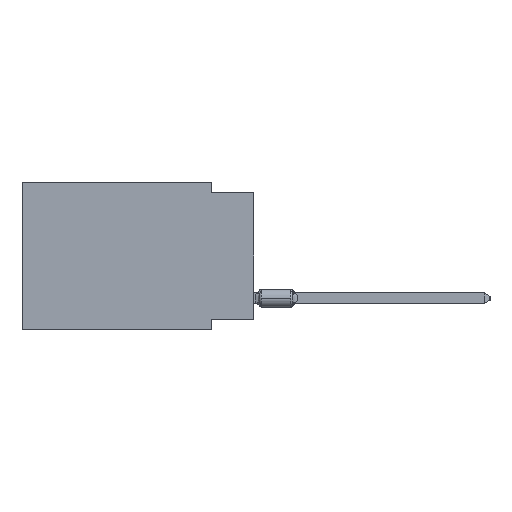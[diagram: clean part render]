
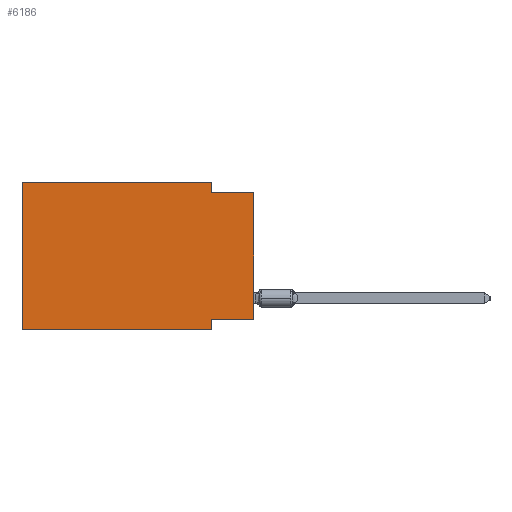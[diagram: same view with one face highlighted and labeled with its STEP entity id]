
A CAD part, left-side view. The second image highlights one B-rep face of the part: STEP entity #6186.
In plain terms, the highlighted planar face has unit normal (-1, 0, 0).
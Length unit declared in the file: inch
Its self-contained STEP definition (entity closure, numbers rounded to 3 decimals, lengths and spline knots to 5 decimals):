
#2592 = CARTESIAN_POINT ( 'NONE',  ( 0., 0.1, 0. ) ) ;
#2606 = ORIENTED_EDGE ( 'NONE', *, *, #16428, .T. ) ;
#2696 = EDGE_LOOP ( 'NONE', ( #2606, #30905, #3369, #40720, #10590, #12407, #20386, #7470 ) ) ;
#2718 = CARTESIAN_POINT ( 'NONE',  ( 0., 0.55, 0. ) ) ;
#2725 = VERTEX_POINT ( 'NONE', #41874 ) ;
#3369 = ORIENTED_EDGE ( 'NONE', *, *, #33779, .F. ) ;
#3439 = CARTESIAN_POINT ( 'NONE',  ( 0., 0., -0.325 ) ) ;
#3729 = CARTESIAN_POINT ( 'NONE',  ( 0., 0.55, 0. ) ) ;
#4168 = CARTESIAN_POINT ( 'NONE',  ( 0., 0.55, 0. ) ) ;
#6186 = ADVANCED_FACE ( 'NONE', ( #16528 ), #30312, .F. ) ;
#7351 = DIRECTION ( 'NONE',  ( 1., 0., 0. ) ) ;
#7470 = ORIENTED_EDGE ( 'NONE', *, *, #14924, .F. ) ;
#8074 = VERTEX_POINT ( 'NONE', #2592 ) ;
#10346 = DIRECTION ( 'NONE',  ( 0., 0., -1. ) ) ;
#10590 = ORIENTED_EDGE ( 'NONE', *, *, #40775, .F. ) ;
#11443 = DIRECTION ( 'NONE',  ( 0., -1., 0. ) ) ;
#11640 = VECTOR ( 'NONE', #35230, 39.37008 ) ;
#12407 = ORIENTED_EDGE ( 'NONE', *, *, #34092, .T. ) ;
#13133 = CARTESIAN_POINT ( 'NONE',  ( 0., 0.1, -0.35 ) ) ;
#14039 = CARTESIAN_POINT ( 'NONE',  ( 0., 0.55, -0.35 ) ) ;
#14924 = EDGE_CURVE ( 'NONE', #16564, #36497, #29581, .T. ) ;
#16428 = EDGE_CURVE ( 'NONE', #16564, #35819, #33630, .T. ) ;
#16528 = FACE_OUTER_BOUND ( 'NONE', #2696, .T. ) ;
#16564 = VERTEX_POINT ( 'NONE', #39547 ) ;
#19637 = CARTESIAN_POINT ( 'NONE',  ( 0., 0.1, -0.325 ) ) ;
#20103 = DIRECTION ( 'NONE',  ( 0., -1., 0. ) ) ;
#20386 = ORIENTED_EDGE ( 'NONE', *, *, #22938, .F. ) ;
#21059 = DIRECTION ( 'NONE',  ( 0., 0., 1. ) ) ;
#21420 = LINE ( 'NONE', #27385, #25381 ) ;
#22938 = EDGE_CURVE ( 'NONE', #36497, #23131, #41605, .T. ) ;
#23131 = VERTEX_POINT ( 'NONE', #13133 ) ;
#24572 = VECTOR ( 'NONE', #21059, 39.37008 ) ;
#24679 = LINE ( 'NONE', #34054, #29037 ) ;
#25001 = DIRECTION ( 'NONE',  ( 0., 0., 1. ) ) ;
#25381 = VECTOR ( 'NONE', #11443, 39.37008 ) ;
#25797 = VERTEX_POINT ( 'NONE', #33505 ) ;
#25821 = VECTOR ( 'NONE', #30204, 39.37008 ) ;
#26992 = DIRECTION ( 'NONE',  ( 0., -1., 0. ) ) ;
#27015 = AXIS2_PLACEMENT_3D ( 'NONE', #4168, #7351, #10346 ) ;
#27094 = LINE ( 'NONE', #3729, #41426 ) ;
#27373 = CARTESIAN_POINT ( 'NONE',  ( 0., 0., -0.025 ) ) ;
#27385 = CARTESIAN_POINT ( 'NONE',  ( 0., 0., -0.025 ) ) ;
#27661 = DIRECTION ( 'NONE',  ( 0., 0., -1. ) ) ;
#28202 = LINE ( 'NONE', #41169, #29539 ) ;
#29037 = VECTOR ( 'NONE', #27661, 39.37008 ) ;
#29539 = VECTOR ( 'NONE', #25001, 39.37008 ) ;
#29581 = LINE ( 'NONE', #3439, #25821 ) ;
#29612 = EDGE_CURVE ( 'NONE', #2725, #35819, #21420, .T. ) ;
#30187 = LINE ( 'NONE', #14039, #37876 ) ;
#30204 = DIRECTION ( 'NONE',  ( 0., 1., 0. ) ) ;
#30312 = PLANE ( 'NONE',  #27015 ) ;
#30622 = CARTESIAN_POINT ( 'NONE',  ( 0., 0., 0. ) ) ;
#30905 = ORIENTED_EDGE ( 'NONE', *, *, #29612, .F. ) ;
#33505 = CARTESIAN_POINT ( 'NONE',  ( 0., 0.55, -0.35 ) ) ;
#33630 = LINE ( 'NONE', #30622, #24572 ) ;
#33779 = EDGE_CURVE ( 'NONE', #8074, #2725, #24679, .T. ) ;
#34054 = CARTESIAN_POINT ( 'NONE',  ( 0., 0.1, 0. ) ) ;
#34092 = EDGE_CURVE ( 'NONE', #25797, #23131, #30187, .T. ) ;
#35230 = DIRECTION ( 'NONE',  ( 0., 0., -1. ) ) ;
#35452 = CARTESIAN_POINT ( 'NONE',  ( 0., 0.1, -0.35 ) ) ;
#35819 = VERTEX_POINT ( 'NONE', #27373 ) ;
#36497 = VERTEX_POINT ( 'NONE', #19637 ) ;
#37132 = VERTEX_POINT ( 'NONE', #2718 ) ;
#37876 = VECTOR ( 'NONE', #26992, 39.37008 ) ;
#38571 = EDGE_CURVE ( 'NONE', #37132, #8074, #27094, .T. ) ;
#39547 = CARTESIAN_POINT ( 'NONE',  ( 0., 0., -0.325 ) ) ;
#40720 = ORIENTED_EDGE ( 'NONE', *, *, #38571, .F. ) ;
#40775 = EDGE_CURVE ( 'NONE', #25797, #37132, #28202, .T. ) ;
#41169 = CARTESIAN_POINT ( 'NONE',  ( 0., 0.55, 0. ) ) ;
#41426 = VECTOR ( 'NONE', #20103, 39.37008 ) ;
#41605 = LINE ( 'NONE', #35452, #11640 ) ;
#41874 = CARTESIAN_POINT ( 'NONE',  ( 0., 0.1, -0.025 ) ) ;
